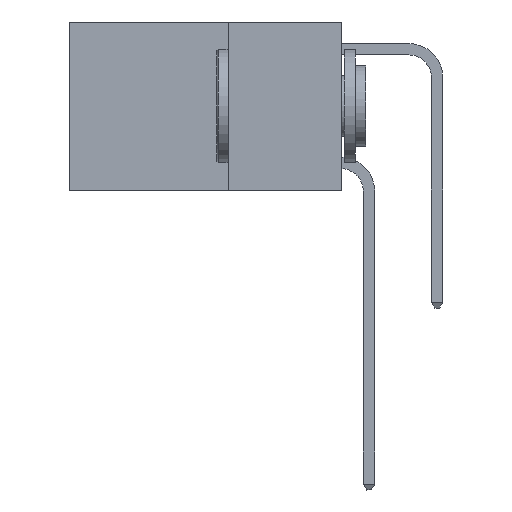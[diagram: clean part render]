
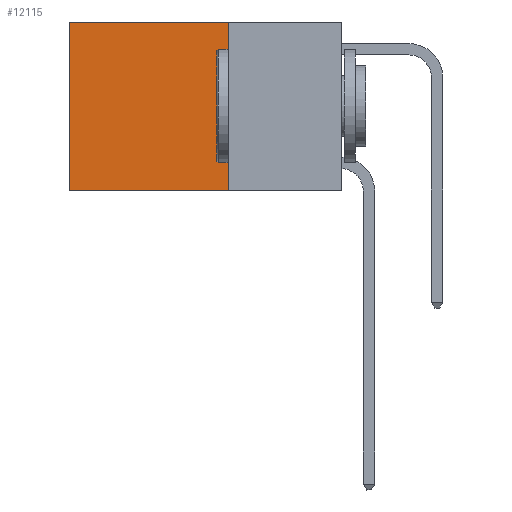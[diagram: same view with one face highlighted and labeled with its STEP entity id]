
A CAD part, left-side view. The second image highlights one B-rep face of the part: STEP entity #12115.
In plain terms, the highlighted planar face has unit normal (-1, 0, 0).
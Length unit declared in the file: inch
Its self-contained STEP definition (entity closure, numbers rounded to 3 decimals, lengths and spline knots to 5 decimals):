
#463 = ORIENTED_EDGE ( 'NONE', *, *, #13395, .F. ) ;
#2147 = CARTESIAN_POINT ( 'NONE',  ( 0.2625, 0.25, -0.37 ) ) ;
#2344 = EDGE_CURVE ( 'NONE', #14429, #11639, #9440, .T. ) ;
#4266 = PLANE ( 'NONE',  #20379 ) ;
#4344 = ORIENTED_EDGE ( 'NONE', *, *, #7438, .T. ) ;
#5498 = CARTESIAN_POINT ( 'NONE',  ( 0.2625, 0.25, 0. ) ) ;
#5537 = CARTESIAN_POINT ( 'NONE',  ( 0.2625, 0.25, 0. ) ) ;
#5746 = VECTOR ( 'NONE', #14793, 39.37008 ) ;
#6221 = DIRECTION ( 'NONE',  ( 0., 1., 0. ) ) ;
#6299 = ORIENTED_EDGE ( 'NONE', *, *, #6361, .T. ) ;
#6361 = EDGE_CURVE ( 'NONE', #16113, #7098, #12774, .T. ) ;
#6766 = CARTESIAN_POINT ( 'NONE',  ( 0.2625, 0.6, -0.37 ) ) ;
#7098 = VERTEX_POINT ( 'NONE', #6766 ) ;
#7438 = EDGE_CURVE ( 'NONE', #14429, #16113, #12702, .T. ) ;
#7820 = CARTESIAN_POINT ( 'NONE',  ( 0.2625, 0.6, 0. ) ) ;
#7945 = CARTESIAN_POINT ( 'NONE',  ( 0.2625, 0.25, 0. ) ) ;
#9065 = DIRECTION ( 'NONE',  ( 0., 0., -1. ) ) ;
#9265 = CARTESIAN_POINT ( 'NONE',  ( 0.2625, 0.6, 0. ) ) ;
#9440 = LINE ( 'NONE', #7945, #19882 ) ;
#10862 = DIRECTION ( 'NONE',  ( 1., 0., 0. ) ) ;
#11639 = VERTEX_POINT ( 'NONE', #11731 ) ;
#11731 = CARTESIAN_POINT ( 'NONE',  ( 0.2625, 0.25, -0.37 ) ) ;
#12115 = ADVANCED_FACE ( 'NONE', ( #20214 ), #4266, .F. ) ;
#12664 = DIRECTION ( 'NONE',  ( 0., 0., -1. ) ) ;
#12702 = LINE ( 'NONE', #20456, #14690 ) ;
#12774 = LINE ( 'NONE', #9265, #19124 ) ;
#12960 = EDGE_LOOP ( 'NONE', ( #6299, #463, #13935, #4344 ) ) ;
#13395 = EDGE_CURVE ( 'NONE', #11639, #7098, #19683, .T. ) ;
#13935 = ORIENTED_EDGE ( 'NONE', *, *, #2344, .F. ) ;
#14429 = VERTEX_POINT ( 'NONE', #5498 ) ;
#14690 = VECTOR ( 'NONE', #6221, 39.37008 ) ;
#14793 = DIRECTION ( 'NONE',  ( 0., 1., 0. ) ) ;
#16113 = VERTEX_POINT ( 'NONE', #7820 ) ;
#19124 = VECTOR ( 'NONE', #12664, 39.37008 ) ;
#19683 = LINE ( 'NONE', #2147, #5746 ) ;
#19882 = VECTOR ( 'NONE', #20899, 39.37008 ) ;
#20214 = FACE_OUTER_BOUND ( 'NONE', #12960, .T. ) ;
#20379 = AXIS2_PLACEMENT_3D ( 'NONE', #5537, #10862, #9065 ) ;
#20456 = CARTESIAN_POINT ( 'NONE',  ( 0.2625, 0.25, 0. ) ) ;
#20899 = DIRECTION ( 'NONE',  ( 0., 0., -1. ) ) ;
